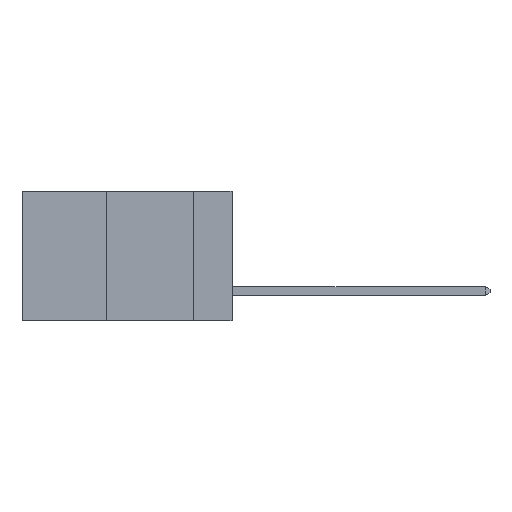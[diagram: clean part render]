
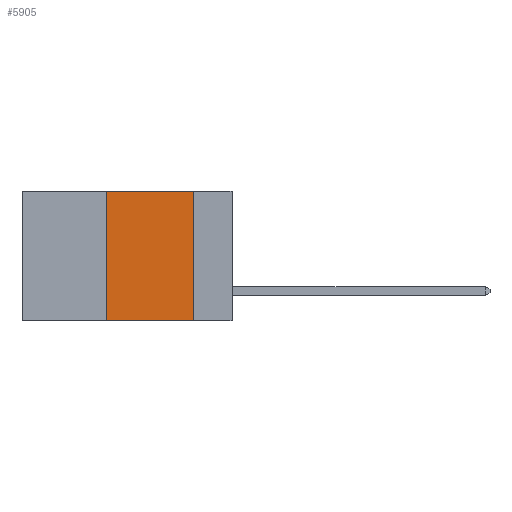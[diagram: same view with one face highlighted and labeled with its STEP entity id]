
A CAD part, left-side view. The second image highlights one B-rep face of the part: STEP entity #5905.
In plain terms, the highlighted planar face has unit normal (-1, 0, 0).
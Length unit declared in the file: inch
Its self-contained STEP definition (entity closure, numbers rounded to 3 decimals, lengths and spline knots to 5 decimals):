
#1537 = ORIENTED_EDGE ( 'NONE', *, *, #13538, .F. ) ;
#1695 = VECTOR ( 'NONE', #9113, 39.37008 ) ;
#2187 = ORIENTED_EDGE ( 'NONE', *, *, #7007, .F. ) ;
#2885 = CARTESIAN_POINT ( 'NONE',  ( 0., 0.11, 0. ) ) ;
#3667 = LINE ( 'NONE', #12697, #12035 ) ;
#4057 = LINE ( 'NONE', #11628, #11918 ) ;
#4084 = EDGE_CURVE ( 'NONE', #14329, #14370, #4057, .T. ) ;
#4398 = VERTEX_POINT ( 'NONE', #13847 ) ;
#4692 = ORIENTED_EDGE ( 'NONE', *, *, #4084, .T. ) ;
#5682 = VECTOR ( 'NONE', #8829, 39.37008 ) ;
#5905 = ADVANCED_FACE ( 'NONE', ( #7695 ), #16379, .F. ) ;
#7007 = EDGE_CURVE ( 'NONE', #4398, #19380, #3667, .T. ) ;
#7036 = CARTESIAN_POINT ( 'NONE',  ( 0., 0.6, 0. ) ) ;
#7298 = EDGE_CURVE ( 'NONE', #14329, #4398, #18134, .T. ) ;
#7558 = CARTESIAN_POINT ( 'NONE',  ( 0., 0.11, 0. ) ) ;
#7695 = FACE_OUTER_BOUND ( 'NONE', #19449, .T. ) ;
#8594 = DIRECTION ( 'NONE',  ( 1., 0., 0. ) ) ;
#8829 = DIRECTION ( 'NONE',  ( 0., 0., 1. ) ) ;
#9113 = DIRECTION ( 'NONE',  ( 0., 0., -1. ) ) ;
#11628 = CARTESIAN_POINT ( 'NONE',  ( 0., 0.6, -0.37 ) ) ;
#11918 = VECTOR ( 'NONE', #13188, 39.37008 ) ;
#12035 = VECTOR ( 'NONE', #17417, 39.37008 ) ;
#12697 = CARTESIAN_POINT ( 'NONE',  ( 0., 0.6, 0. ) ) ;
#13188 = DIRECTION ( 'NONE',  ( 0., -1., 0. ) ) ;
#13451 = CARTESIAN_POINT ( 'NONE',  ( 0., 0.36, 0. ) ) ;
#13538 = EDGE_CURVE ( 'NONE', #19380, #14370, #14279, .T. ) ;
#13847 = CARTESIAN_POINT ( 'NONE',  ( 0., 0.36, 0. ) ) ;
#14279 = LINE ( 'NONE', #7558, #1695 ) ;
#14329 = VERTEX_POINT ( 'NONE', #14392 ) ;
#14370 = VERTEX_POINT ( 'NONE', #19172 ) ;
#14392 = CARTESIAN_POINT ( 'NONE',  ( 0., 0.36, -0.37 ) ) ;
#16379 = PLANE ( 'NONE',  #17291 ) ;
#17163 = ORIENTED_EDGE ( 'NONE', *, *, #7298, .F. ) ;
#17291 = AXIS2_PLACEMENT_3D ( 'NONE', #7036, #8594, #19505 ) ;
#17417 = DIRECTION ( 'NONE',  ( 0., -1., 0. ) ) ;
#18134 = LINE ( 'NONE', #13451, #5682 ) ;
#19172 = CARTESIAN_POINT ( 'NONE',  ( 0., 0.11, -0.37 ) ) ;
#19380 = VERTEX_POINT ( 'NONE', #2885 ) ;
#19449 = EDGE_LOOP ( 'NONE', ( #1537, #2187, #17163, #4692 ) ) ;
#19505 = DIRECTION ( 'NONE',  ( 0., 0., -1. ) ) ;
